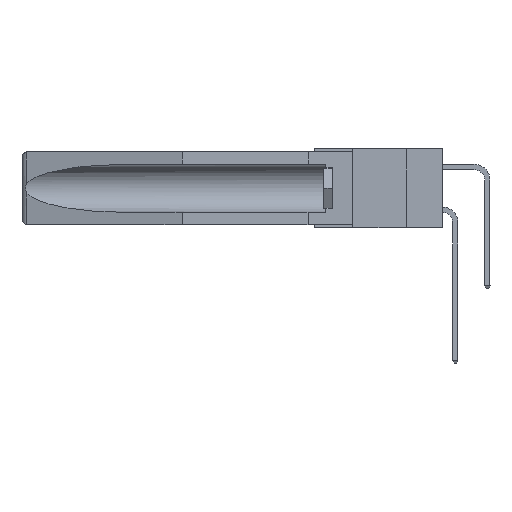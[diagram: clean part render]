
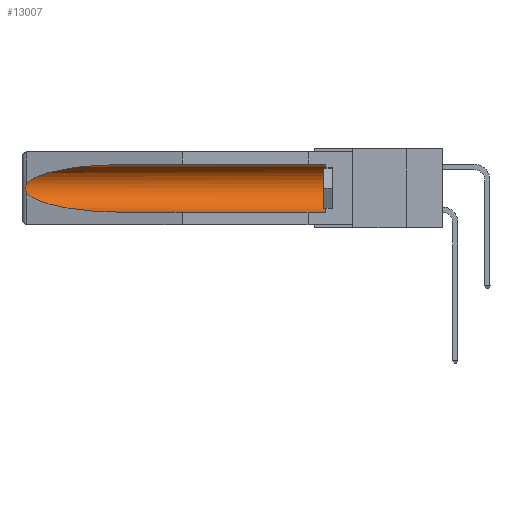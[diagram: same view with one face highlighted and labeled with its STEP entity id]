
A CAD part, left-side view. The second image highlights one B-rep face of the part: STEP entity #13007.
In plain terms, the highlighted cylindrical face has radius 2.857 mm (diameter 5.715 mm), a partial arc.
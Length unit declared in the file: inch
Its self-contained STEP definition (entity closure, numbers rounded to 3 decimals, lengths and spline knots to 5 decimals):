
#18 = EDGE_CURVE ( 'NONE', #8753, #14181, #31893, .T. ) ;
#25 = LINE ( 'NONE', #27029, #9238 ) ;
#254 = CARTESIAN_POINT ( 'NONE',  ( 0.2673, 1.5327, -0.16383 ) ) ;
#403 = EDGE_CURVE ( 'NONE', #21726, #1616, #3259, .T. ) ;
#409 = ORIENTED_EDGE ( 'NONE', *, *, #29562, .T. ) ;
#978 = B_SPLINE_CURVE_WITH_KNOTS ( 'NONE', 3,
 ( #21607, #3890, #2624, #254, #20443, #5214, #7884, #27949, #32974, #28167 ),
 .UNSPECIFIED., .F., .F.,
 ( 4, 2, 2, 2, 4 ),
 ( 0., 0.00029, 0.00058, 0.00087, 0.00117 ),
 .UNSPECIFIED. ) ;
#1616 = VERTEX_POINT ( 'NONE', #23197 ) ;
#2306 = DIRECTION ( 'NONE',  ( 0., 0., 1. ) ) ;
#2459 = DIRECTION ( 'NONE',  ( 0., -1., 0. ) ) ;
#2567 = CARTESIAN_POINT ( 'NONE',  ( 0.21114, 1.30732, -0.059 ) ) ;
#2624 = CARTESIAN_POINT ( 'NONE',  ( 0.26654, 1.53092, -0.15636 ) ) ;
#3259 =( BOUNDED_CURVE ( )  B_SPLINE_CURVE ( 3, ( #23206, #2567, #18159, #5164 ),
 .UNSPECIFIED., .F., .F. ) 
 B_SPLINE_CURVE_WITH_KNOTS ( ( 4, 4 ),
 ( 4.71239, 6.08839 ),
 .UNSPECIFIED. ) 
 CURVE ( )  GEOMETRIC_REPRESENTATION_ITEM ( )  RATIONAL_B_SPLINE_CURVE ( ( 1., 0.848, 0.848, 1. ) ) 
 REPRESENTATION_ITEM ( '' )  );
#3890 = CARTESIAN_POINT ( 'NONE',  ( 0.26597, 1.52961, -0.15275 ) ) ;
#4785 = DIRECTION ( 'NONE',  ( 0., 1., 0. ) ) ;
#5164 = CARTESIAN_POINT ( 'NONE',  ( 0.26537, 1.52718, -0.14972 ) ) ;
#5214 = CARTESIAN_POINT ( 'NONE',  ( 0.2675, 1.53308, -0.17534 ) ) ;
#5810 = DIRECTION ( 'NONE',  ( 0., 1., 0. ) ) ;
#6857 = CARTESIAN_POINT ( 'NONE',  ( 0.155, 1.07973, -0.284 ) ) ;
#7262 = AXIS2_PLACEMENT_3D ( 'NONE', #7801, #4785, #2306 ) ;
#7801 = CARTESIAN_POINT ( 'NONE',  ( 0.155, -0.30754, -0.1715 ) ) ;
#7884 = CARTESIAN_POINT ( 'NONE',  ( 0.2673, 1.53269, -0.17917 ) ) ;
#8266 = CARTESIAN_POINT ( 'NONE',  ( 0.155, -0.30754, -0.059 ) ) ;
#8753 = VERTEX_POINT ( 'NONE', #31784 ) ;
#9238 = VECTOR ( 'NONE', #23960, 39.37008 ) ;
#10619 = ORIENTED_EDGE ( 'NONE', *, *, #22227, .T. ) ;
#12004 = EDGE_CURVE ( 'NONE', #27181, #23196, #23326, .T. ) ;
#13007 = ADVANCED_FACE ( 'NONE', ( #15659 ), #20043, .F. ) ;
#13245 = EDGE_LOOP ( 'NONE', ( #22200, #10619, #19092, #31788, #27200, #409 ) ) ;
#14181 = VERTEX_POINT ( 'NONE', #6857 ) ;
#14622 = CARTESIAN_POINT ( 'NONE',  ( 0.155, 0.126, -0.284 ) ) ;
#15627 = LINE ( 'NONE', #8266, #19999 ) ;
#15659 = FACE_OUTER_BOUND ( 'NONE', #13245, .T. ) ;
#16469 = CARTESIAN_POINT ( 'NONE',  ( 0.155, 1.07973, -0.059 ) ) ;
#18159 = CARTESIAN_POINT ( 'NONE',  ( 0.25451, 1.48313, -0.09465 ) ) ;
#18299 = CARTESIAN_POINT ( 'NONE',  ( 0.155, 1.07973, -0.284 ) ) ;
#19092 = ORIENTED_EDGE ( 'NONE', *, *, #18, .T. ) ;
#19999 = VECTOR ( 'NONE', #5810, 39.37008 ) ;
#20043 = CYLINDRICAL_SURFACE ( 'NONE', #7262, 0.1125 ) ;
#20443 = CARTESIAN_POINT ( 'NONE',  ( 0.2675, 1.53308, -0.16763 ) ) ;
#21067 = AXIS2_PLACEMENT_3D ( 'NONE', #25189, #2459, #27876 ) ;
#21070 = CARTESIAN_POINT ( 'NONE',  ( 0.25451, 1.48313, -0.24835 ) ) ;
#21607 = CARTESIAN_POINT ( 'NONE',  ( 0.26537, 1.52718, -0.14972 ) ) ;
#21726 = VERTEX_POINT ( 'NONE', #16469 ) ;
#22059 = CARTESIAN_POINT ( 'NONE',  ( 0.155, 0.126, -0.059 ) ) ;
#22200 = ORIENTED_EDGE ( 'NONE', *, *, #403, .T. ) ;
#22227 = EDGE_CURVE ( 'NONE', #1616, #8753, #978, .T. ) ;
#23196 = VERTEX_POINT ( 'NONE', #22059 ) ;
#23197 = CARTESIAN_POINT ( 'NONE',  ( 0.26537, 1.52718, -0.14972 ) ) ;
#23206 = CARTESIAN_POINT ( 'NONE',  ( 0.155, 1.07973, -0.059 ) ) ;
#23244 = CARTESIAN_POINT ( 'NONE',  ( 0.26537, 1.52718, -0.19328 ) ) ;
#23326 = CIRCLE ( 'NONE', #21067, 0.1125 ) ;
#23960 = DIRECTION ( 'NONE',  ( 0., 1., 0. ) ) ;
#25189 = CARTESIAN_POINT ( 'NONE',  ( 0.155, 0.126, -0.1715 ) ) ;
#27029 = CARTESIAN_POINT ( 'NONE',  ( 0.155, -0.30754, -0.284 ) ) ;
#27181 = VERTEX_POINT ( 'NONE', #14622 ) ;
#27200 = ORIENTED_EDGE ( 'NONE', *, *, #12004, .T. ) ;
#27876 = DIRECTION ( 'NONE',  ( 0., 0., 1. ) ) ;
#27949 = CARTESIAN_POINT ( 'NONE',  ( 0.26655, 1.53094, -0.18657 ) ) ;
#28167 = CARTESIAN_POINT ( 'NONE',  ( 0.26537, 1.52718, -0.19328 ) ) ;
#28357 = CARTESIAN_POINT ( 'NONE',  ( 0.21114, 1.30732, -0.284 ) ) ;
#29562 = EDGE_CURVE ( 'NONE', #23196, #21726, #15627, .T. ) ;
#29713 = EDGE_CURVE ( 'NONE', #27181, #14181, #25, .T. ) ;
#31784 = CARTESIAN_POINT ( 'NONE',  ( 0.26537, 1.52718, -0.19328 ) ) ;
#31788 = ORIENTED_EDGE ( 'NONE', *, *, #29713, .F. ) ;
#31893 =( BOUNDED_CURVE ( )  B_SPLINE_CURVE ( 3, ( #23244, #21070, #28357, #18299 ),
 .UNSPECIFIED., .F., .T. ) 
 B_SPLINE_CURVE_WITH_KNOTS ( ( 4, 4 ),
 ( 0.1948, 1.5708 ),
 .UNSPECIFIED. ) 
 CURVE ( )  GEOMETRIC_REPRESENTATION_ITEM ( )  RATIONAL_B_SPLINE_CURVE ( ( 1., 0.848, 0.848, 1. ) ) 
 REPRESENTATION_ITEM ( '' )  );
#32974 = CARTESIAN_POINT ( 'NONE',  ( 0.26597, 1.5296, -0.19026 ) ) ;
